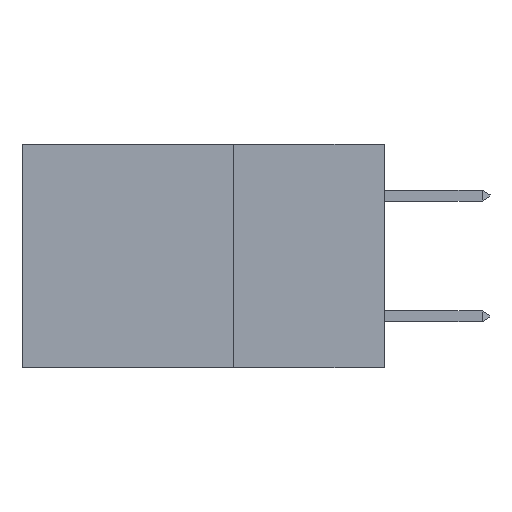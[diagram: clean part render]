
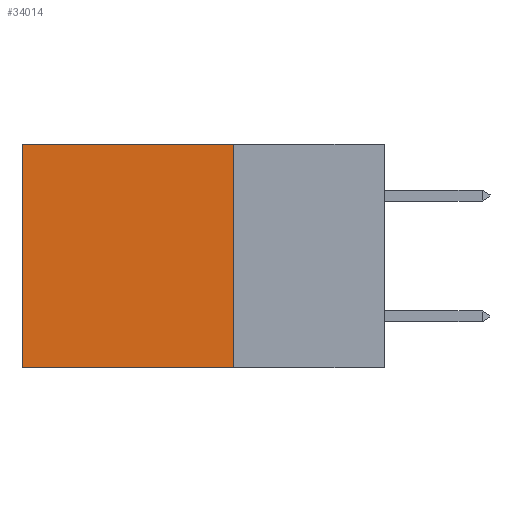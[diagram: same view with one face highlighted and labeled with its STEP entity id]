
A CAD part, left-side view. The second image highlights one B-rep face of the part: STEP entity #34014.
In plain terms, the highlighted planar face has unit normal (-1, 0, 0).
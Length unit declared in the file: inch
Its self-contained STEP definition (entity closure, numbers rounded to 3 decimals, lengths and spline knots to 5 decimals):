
#2114 = EDGE_LOOP ( 'NONE', ( #10079, #17908, #33074, #21679 ) ) ;
#3455 = VERTEX_POINT ( 'NONE', #12297 ) ;
#3670 = CARTESIAN_POINT ( 'NONE',  ( 0.2875, 0.25, -0.37 ) ) ;
#5029 = FACE_OUTER_BOUND ( 'NONE', #2114, .T. ) ;
#5962 = CARTESIAN_POINT ( 'NONE',  ( 0.2875, 0.25, 0. ) ) ;
#9196 = AXIS2_PLACEMENT_3D ( 'NONE', #14156, #30941, #23719 ) ;
#9567 = DIRECTION ( 'NONE',  ( 0., 0., -1. ) ) ;
#9568 = LINE ( 'NONE', #5962, #23364 ) ;
#10057 = EDGE_CURVE ( 'NONE', #25080, #3455, #12180, .T. ) ;
#10079 = ORIENTED_EDGE ( 'NONE', *, *, #16451, .T. ) ;
#12180 = LINE ( 'NONE', #41103, #15610 ) ;
#12297 = CARTESIAN_POINT ( 'NONE',  ( 0.2875, 0.6, -0.37 ) ) ;
#12744 = LINE ( 'NONE', #35489, #38774 ) ;
#14156 = CARTESIAN_POINT ( 'NONE',  ( 0.2875, 0.25, 0. ) ) ;
#15610 = VECTOR ( 'NONE', #21950, 39.37008 ) ;
#16451 = EDGE_CURVE ( 'NONE', #20879, #3455, #12744, .T. ) ;
#17908 = ORIENTED_EDGE ( 'NONE', *, *, #10057, .F. ) ;
#18917 = DIRECTION ( 'NONE',  ( 0., 0., -1. ) ) ;
#20879 = VERTEX_POINT ( 'NONE', #36654 ) ;
#21679 = ORIENTED_EDGE ( 'NONE', *, *, #34197, .T. ) ;
#21950 = DIRECTION ( 'NONE',  ( 0., 1., 0. ) ) ;
#23364 = VECTOR ( 'NONE', #18917, 39.37008 ) ;
#23719 = DIRECTION ( 'NONE',  ( 0., 0., -1. ) ) ;
#25080 = VERTEX_POINT ( 'NONE', #3670 ) ;
#25869 = VERTEX_POINT ( 'NONE', #33985 ) ;
#29214 = CARTESIAN_POINT ( 'NONE',  ( 0.2875, 0.25, 0. ) ) ;
#30311 = PLANE ( 'NONE',  #9196 ) ;
#30941 = DIRECTION ( 'NONE',  ( 1., 0., 0. ) ) ;
#31252 = EDGE_CURVE ( 'NONE', #25869, #25080, #9568, .T. ) ;
#33030 = LINE ( 'NONE', #29214, #36346 ) ;
#33074 = ORIENTED_EDGE ( 'NONE', *, *, #31252, .F. ) ;
#33985 = CARTESIAN_POINT ( 'NONE',  ( 0.2875, 0.25, 0. ) ) ;
#34014 = ADVANCED_FACE ( 'NONE', ( #5029 ), #30311, .F. ) ;
#34197 = EDGE_CURVE ( 'NONE', #25869, #20879, #33030, .T. ) ;
#35489 = CARTESIAN_POINT ( 'NONE',  ( 0.2875, 0.6, 0. ) ) ;
#35789 = DIRECTION ( 'NONE',  ( 0., 1., 0. ) ) ;
#36346 = VECTOR ( 'NONE', #35789, 39.37008 ) ;
#36654 = CARTESIAN_POINT ( 'NONE',  ( 0.2875, 0.6, 0. ) ) ;
#38774 = VECTOR ( 'NONE', #9567, 39.37008 ) ;
#41103 = CARTESIAN_POINT ( 'NONE',  ( 0.2875, 0.25, -0.37 ) ) ;
